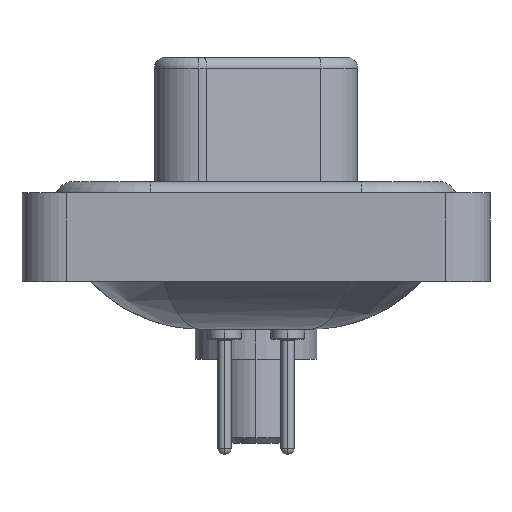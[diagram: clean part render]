
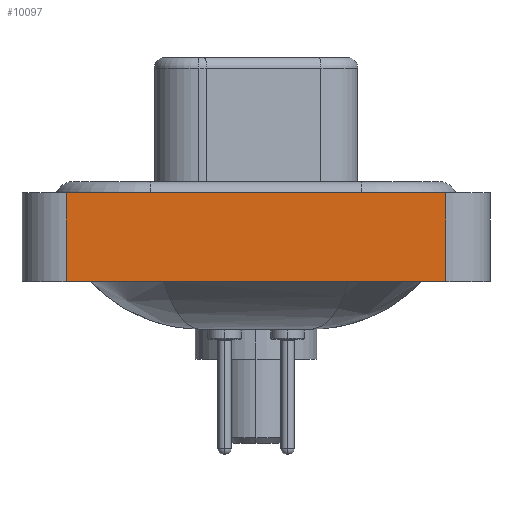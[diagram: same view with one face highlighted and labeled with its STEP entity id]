
A CAD part, left-side view. The second image highlights one B-rep face of the part: STEP entity #10097.
In plain terms, the highlighted planar face has unit normal (-1, 0, 0).
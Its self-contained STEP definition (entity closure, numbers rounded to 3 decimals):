
#359 = VERTEX_POINT ( 'NONE', #10891 ) ;
#409 = EDGE_CURVE ( 'NONE', #18473, #18297, #7762, .T. ) ;
#571 = CARTESIAN_POINT ( 'NONE',  ( -7.3, -8.55, -3.6 ) ) ;
#657 = ORIENTED_EDGE ( 'NONE', *, *, #18215, .F. ) ;
#673 = DIRECTION ( 'NONE',  ( 0., -1., 0. ) ) ;
#2092 = EDGE_CURVE ( 'NONE', #18473, #10842, #4914, .T. ) ;
#2693 = LINE ( 'NONE', #17079, #19026 ) ;
#3356 = DIRECTION ( 'NONE',  ( -1., 0., 0. ) ) ;
#3822 = CARTESIAN_POINT ( 'NONE',  ( -7.3, -8.55, 0.4 ) ) ;
#4914 = LINE ( 'NONE', #12804, #13427 ) ;
#5536 = CARTESIAN_POINT ( 'NONE',  ( -7.3, 8.55, 0.4 ) ) ;
#7265 = EDGE_CURVE ( 'NONE', #18297, #359, #2693, .T. ) ;
#7762 = LINE ( 'NONE', #19879, #14643 ) ;
#8144 = CARTESIAN_POINT ( 'NONE',  ( -7.3, -8.55, -3.6 ) ) ;
#8604 = VECTOR ( 'NONE', #673, 1000. ) ;
#8747 = AXIS2_PLACEMENT_3D ( 'NONE', #8144, #3356, #11285 ) ;
#10097 = ADVANCED_FACE ( 'NONE', ( #17545 ), #18891, .T. ) ;
#10842 = VERTEX_POINT ( 'NONE', #5536 ) ;
#10891 = CARTESIAN_POINT ( 'NONE',  ( -7.3, -8.55, 0.4 ) ) ;
#10975 = ORIENTED_EDGE ( 'NONE', *, *, #2092, .F. ) ;
#11285 = DIRECTION ( 'NONE',  ( 0., 0., 1. ) ) ;
#12353 = CARTESIAN_POINT ( 'NONE',  ( -7.3, 8.55, -3.6 ) ) ;
#12804 = CARTESIAN_POINT ( 'NONE',  ( -7.3, 8.55, -3.6 ) ) ;
#13427 = VECTOR ( 'NONE', #14272, 1000. ) ;
#13634 = DIRECTION ( 'NONE',  ( 0., -1., 0. ) ) ;
#13747 = DIRECTION ( 'NONE',  ( 0., 0., 1. ) ) ;
#14272 = DIRECTION ( 'NONE',  ( 0., 0., 1. ) ) ;
#14406 = ORIENTED_EDGE ( 'NONE', *, *, #7265, .T. ) ;
#14643 = VECTOR ( 'NONE', #13634, 1000. ) ;
#14857 = LINE ( 'NONE', #3822, #8604 ) ;
#16271 = ORIENTED_EDGE ( 'NONE', *, *, #409, .T. ) ;
#17079 = CARTESIAN_POINT ( 'NONE',  ( -7.3, -8.55, -3.6 ) ) ;
#17545 = FACE_OUTER_BOUND ( 'NONE', #19580, .T. ) ;
#18215 = EDGE_CURVE ( 'NONE', #10842, #359, #14857, .T. ) ;
#18297 = VERTEX_POINT ( 'NONE', #571 ) ;
#18473 = VERTEX_POINT ( 'NONE', #12353 ) ;
#18891 = PLANE ( 'NONE',  #8747 ) ;
#19026 = VECTOR ( 'NONE', #13747, 1000. ) ;
#19580 = EDGE_LOOP ( 'NONE', ( #14406, #657, #10975, #16271 ) ) ;
#19879 = CARTESIAN_POINT ( 'NONE',  ( -7.3, -8.55, -3.6 ) ) ;
